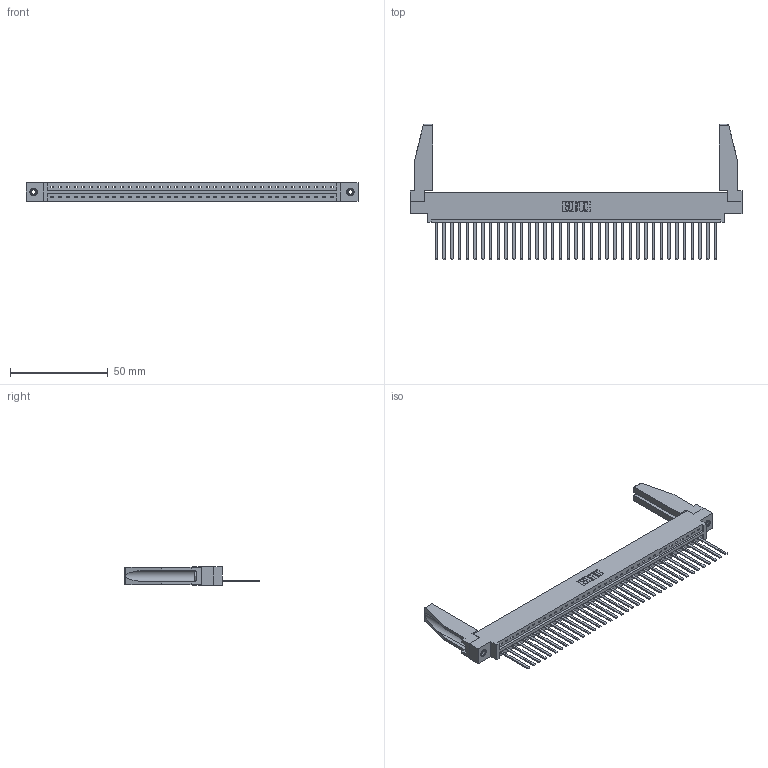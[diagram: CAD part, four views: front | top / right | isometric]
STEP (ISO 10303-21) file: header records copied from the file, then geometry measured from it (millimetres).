
FILE_DESCRIPTION (( 'STEP AP203' ), '1' );
FILE_NAME ('387-037-544-678.STEP', '2019-10-04T15:09:57', ( '' ), ( '' ), 'SwSTEP 2.0', 'SolidWorks 2016', '' );
FILE_SCHEMA (( 'CONFIG_CONTROL_DESIGN' ));
Length unit declared in the file: inch
Products named in the file (5): 345-250-001_345-250-001-102; 337 Part_0.170 Offset - 0.156 Dia-TI; 345-292-001_345-293-144; 387-037-544-678; 307-220-078
Assembly tree (42 placements, depth 2):
  387-037-544-678
    337 Part_0.170 Offset - 0.156 Dia-TI
    345-292-001_345-293-144  x37
    345-250-001_345-250-001-102  x2
    307-220-078  x2
Bounding box: 169.62 x 69.09 x 9.4 mm (x, y, z)
Volume: 21871 mm3; surface area: 23789.1 mm2
Topology: 42 solids, 42 shells, 2320 faces, 6943 edges, 4570 vertices
Faces by surface type: plane 1712, cylinder 592, cone 12, torus 4
Entity records: 30538 total; most frequent: CARTESIAN_POINT 5311, ORIENTED_EDGE 5240, DIRECTION 4486, EDGE_CURVE 2620, VECTOR 2458, LINE 2458, VERTEX_POINT 1740, AXIS2_PLACEMENT_3D 1014
